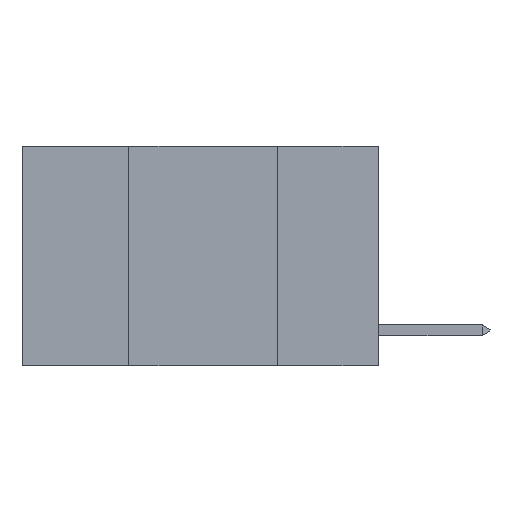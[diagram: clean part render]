
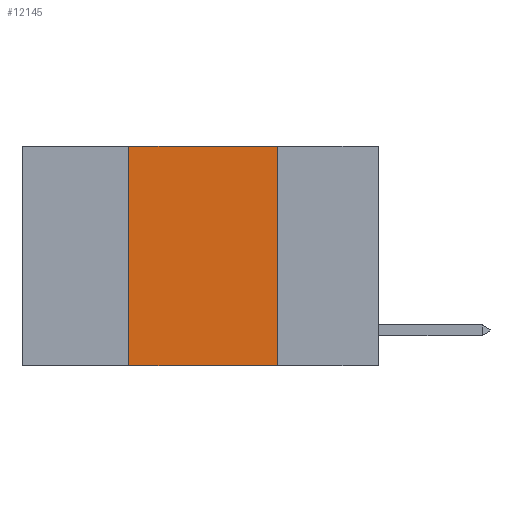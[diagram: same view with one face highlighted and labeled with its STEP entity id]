
A CAD part, left-side view. The second image highlights one B-rep face of the part: STEP entity #12145.
In plain terms, the highlighted planar face has unit normal (-1, 0, 0).
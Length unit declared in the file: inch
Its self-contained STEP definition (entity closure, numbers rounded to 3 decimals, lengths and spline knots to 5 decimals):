
#132 = PLANE ( 'NONE',  #3807 ) ;
#373 = CARTESIAN_POINT ( 'NONE',  ( 0., 0.17, 0. ) ) ;
#501 = DIRECTION ( 'NONE',  ( 0., -1., 0. ) ) ;
#1425 = VECTOR ( 'NONE', #6480, 39.37008 ) ;
#1711 = VERTEX_POINT ( 'NONE', #9656 ) ;
#2043 = ORIENTED_EDGE ( 'NONE', *, *, #4258, .F. ) ;
#2183 = DIRECTION ( 'NONE',  ( 0., 0., 1. ) ) ;
#2361 = ORIENTED_EDGE ( 'NONE', *, *, #4926, .F. ) ;
#2715 = DIRECTION ( 'NONE',  ( 0., 0., -1. ) ) ;
#3031 = CARTESIAN_POINT ( 'NONE',  ( 0., 0.42, 0. ) ) ;
#3571 = VECTOR ( 'NONE', #2183, 39.37008 ) ;
#3807 = AXIS2_PLACEMENT_3D ( 'NONE', #8912, #10137, #2715 ) ;
#4258 = EDGE_CURVE ( 'NONE', #6385, #1711, #12786, .T. ) ;
#4775 = LINE ( 'NONE', #11292, #1425 ) ;
#4926 = EDGE_CURVE ( 'NONE', #10751, #8469, #12245, .T. ) ;
#5783 = CARTESIAN_POINT ( 'NONE',  ( 0., 0.17, -0.37 ) ) ;
#5979 = ORIENTED_EDGE ( 'NONE', *, *, #6517, .T. ) ;
#6006 = VECTOR ( 'NONE', #501, 39.37008 ) ;
#6385 = VERTEX_POINT ( 'NONE', #7750 ) ;
#6480 = DIRECTION ( 'NONE',  ( 0., -1., 0. ) ) ;
#6517 = EDGE_CURVE ( 'NONE', #6385, #8469, #12367, .T. ) ;
#7444 = DIRECTION ( 'NONE',  ( 0., 0., -1. ) ) ;
#7750 = CARTESIAN_POINT ( 'NONE',  ( 0., 0.42, -0.37 ) ) ;
#7896 = CARTESIAN_POINT ( 'NONE',  ( 0., 0.17, 0. ) ) ;
#8469 = VERTEX_POINT ( 'NONE', #5783 ) ;
#8812 = EDGE_CURVE ( 'NONE', #1711, #10751, #4775, .T. ) ;
#8912 = CARTESIAN_POINT ( 'NONE',  ( 0., 0.6, 0. ) ) ;
#9656 = CARTESIAN_POINT ( 'NONE',  ( 0., 0.42, 0. ) ) ;
#10137 = DIRECTION ( 'NONE',  ( 1., 0., 0. ) ) ;
#10751 = VERTEX_POINT ( 'NONE', #373 ) ;
#11292 = CARTESIAN_POINT ( 'NONE',  ( 0., 0.6, 0. ) ) ;
#12007 = FACE_OUTER_BOUND ( 'NONE', #13553, .T. ) ;
#12145 = ADVANCED_FACE ( 'NONE', ( #12007 ), #132, .F. ) ;
#12245 = LINE ( 'NONE', #7896, #15249 ) ;
#12367 = LINE ( 'NONE', #14956, #6006 ) ;
#12786 = LINE ( 'NONE', #3031, #3571 ) ;
#13553 = EDGE_LOOP ( 'NONE', ( #2361, #15283, #2043, #5979 ) ) ;
#14956 = CARTESIAN_POINT ( 'NONE',  ( 0., 0.6, -0.37 ) ) ;
#15249 = VECTOR ( 'NONE', #7444, 39.37008 ) ;
#15283 = ORIENTED_EDGE ( 'NONE', *, *, #8812, .F. ) ;
